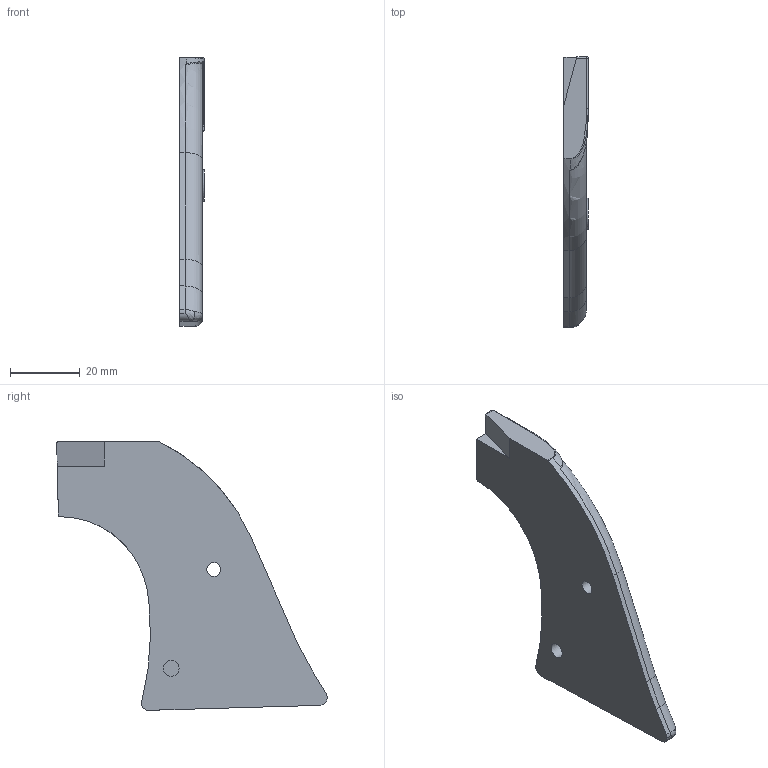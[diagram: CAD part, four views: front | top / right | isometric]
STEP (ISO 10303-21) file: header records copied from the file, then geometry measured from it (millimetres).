
FILE_DESCRIPTION(/* description */ (''),/* implementation_level */ '2;1');
FILE_NAME(/* name */ 'Right Wrangler Slick Grip.step',/* time_stamp */ '2021-09-08T14:28:06-06:00',/* author */ (''),/* organization */ (''),/* preprocessor_version */ 'ST-DEVELOPER v18.1',/* originating_system */ 'Autodesk Translation Framework v10.10.0.1391',/* authorisation */ '');
FILE_SCHEMA (('AUTOMOTIVE_DESIGN { 1 0 10303 214 3 1 1 }'));
Length unit declared in the file: millimetre
Products named in the file (1): Wrangler Mods
Bounding box: 7 x 77.55 x 77 mm (x, y, z)
Volume: 18740.1 mm3; surface area: 8151.8 mm2
Topology: 1 solids, 1 shells, 72 faces, 162 edges, 97 vertices
Faces by surface type: cylinder 31, plane 25, bspline 8, torus 7, sphere 1
Full cylindrical faces by diameter (mm): 4 x1, 4.5 x1, 6.5 x1, 9 x1, 13 x1, 14 x1
Entity records: 2493 total; most frequent: CARTESIAN_POINT 857, DIRECTION 338, ORIENTED_EDGE 324, EDGE_CURVE 162, AXIS2_PLACEMENT_3D 131, VERTEX_POINT 97, EDGE_LOOP 79, LINE 76
